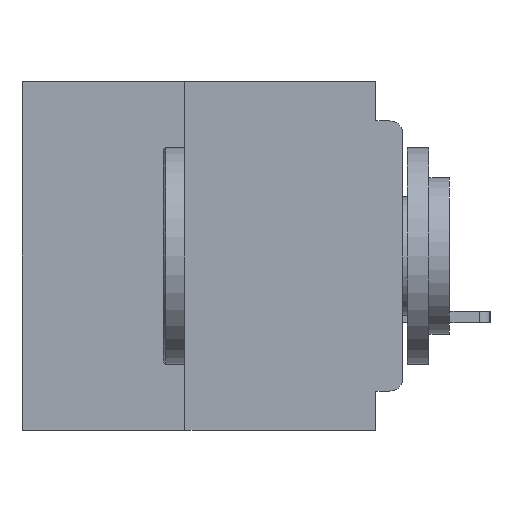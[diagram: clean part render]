
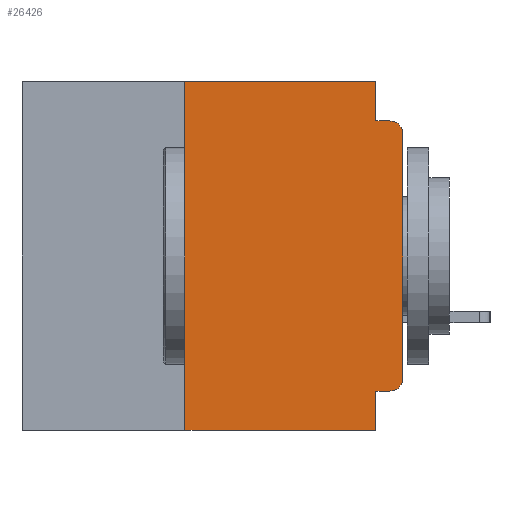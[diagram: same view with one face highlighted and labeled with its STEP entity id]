
A CAD part, left-side view. The second image highlights one B-rep face of the part: STEP entity #26426.
In plain terms, the highlighted planar face has unit normal (-1, 0, 0).
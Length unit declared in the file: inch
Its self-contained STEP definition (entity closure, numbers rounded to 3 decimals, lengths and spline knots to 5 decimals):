
#33 = EDGE_LOOP ( 'NONE', ( #9051, #60994, #26402, #7622, #40816, #59518, #19257, #46271, #60923, #62582 ) ) ;
#771 = DIRECTION ( 'NONE',  ( 0., 0., -1. ) ) ;
#888 = VECTOR ( 'NONE', #58577, 39.37008 ) ;
#1678 = CARTESIAN_POINT ( 'NONE',  ( 0., 0.25, -0.4 ) ) ;
#3356 = DIRECTION ( 'NONE',  ( 0., 1., 0. ) ) ;
#4537 = DIRECTION ( 'NONE',  ( 0., 0., 1. ) ) ;
#5880 = CARTESIAN_POINT ( 'NONE',  ( 0., 0.031, 0. ) ) ;
#7622 = ORIENTED_EDGE ( 'NONE', *, *, #59408, .F. ) ;
#7749 = AXIS2_PLACEMENT_3D ( 'NONE', #62026, #22219, #57303 ) ;
#8075 = VECTOR ( 'NONE', #53399, 39.37008 ) ;
#8453 = CARTESIAN_POINT ( 'NONE',  ( 0., 0.015, -0.045 ) ) ;
#9051 = ORIENTED_EDGE ( 'NONE', *, *, #34646, .T. ) ;
#9626 = VERTEX_POINT ( 'NONE', #39708 ) ;
#11649 = CARTESIAN_POINT ( 'NONE',  ( 0., 0.031, -0.045 ) ) ;
#12040 = PLANE ( 'NONE',  #7749 ) ;
#12617 = VERTEX_POINT ( 'NONE', #48207 ) ;
#12691 = EDGE_CURVE ( 'NONE', #53178, #45963, #41267, .T. ) ;
#13247 = VECTOR ( 'NONE', #771, 39.37008 ) ;
#13794 = CARTESIAN_POINT ( 'NONE',  ( 0., 0.015, -0.06 ) ) ;
#14770 = CARTESIAN_POINT ( 'NONE',  ( 0., 0.25, -0.4 ) ) ;
#16021 = FACE_OUTER_BOUND ( 'NONE', #33, .T. ) ;
#18891 = DIRECTION ( 'NONE',  ( 0., 0., -1. ) ) ;
#19257 = ORIENTED_EDGE ( 'NONE', *, *, #12691, .T. ) ;
#19474 = VERTEX_POINT ( 'NONE', #31330 ) ;
#19723 = DIRECTION ( 'NONE',  ( -1., 0., 0. ) ) ;
#22219 = DIRECTION ( 'NONE',  ( 1., 0., 0. ) ) ;
#22648 = CARTESIAN_POINT ( 'NONE',  ( 0., 0., -0.045 ) ) ;
#22833 = VERTEX_POINT ( 'NONE', #31125 ) ;
#23143 = LINE ( 'NONE', #28608, #34986 ) ;
#23172 = LINE ( 'NONE', #48391, #8075 ) ;
#24656 = LINE ( 'NONE', #22648, #62980 ) ;
#24707 = VERTEX_POINT ( 'NONE', #8453 ) ;
#26339 = CARTESIAN_POINT ( 'NONE',  ( 0., 0., 0. ) ) ;
#26402 = ORIENTED_EDGE ( 'NONE', *, *, #45904, .F. ) ;
#26426 = ADVANCED_FACE ( 'NONE', ( #16021 ), #12040, .F. ) ;
#27227 = CARTESIAN_POINT ( 'NONE',  ( 0., 0., -0.06 ) ) ;
#27704 = EDGE_CURVE ( 'NONE', #39476, #19474, #41979, .T. ) ;
#27709 = DIRECTION ( 'NONE',  ( 0., -1., 0. ) ) ;
#28287 = VECTOR ( 'NONE', #63703, 39.37008 ) ;
#28608 = CARTESIAN_POINT ( 'NONE',  ( 0., 0., -0.355 ) ) ;
#31125 = CARTESIAN_POINT ( 'NONE',  ( 0., 0.031, -0.355 ) ) ;
#31330 = CARTESIAN_POINT ( 'NONE',  ( 0., 0., -0.34 ) ) ;
#33466 = VERTEX_POINT ( 'NONE', #11649 ) ;
#34515 = VECTOR ( 'NONE', #41543, 39.37008 ) ;
#34646 = EDGE_CURVE ( 'NONE', #19474, #50135, #47851, .T. ) ;
#34986 = VECTOR ( 'NONE', #3356, 39.37008 ) ;
#37885 = CARTESIAN_POINT ( 'NONE',  ( 0., 0.031, -0.4 ) ) ;
#39476 = VERTEX_POINT ( 'NONE', #58532 ) ;
#39708 = CARTESIAN_POINT ( 'NONE',  ( 0., 0.25, 0. ) ) ;
#40281 = VECTOR ( 'NONE', #4537, 39.37008 ) ;
#40816 = ORIENTED_EDGE ( 'NONE', *, *, #60432, .F. ) ;
#41267 = LINE ( 'NONE', #53653, #888 ) ;
#41543 = DIRECTION ( 'NONE',  ( 0., 0., 1. ) ) ;
#41979 = CIRCLE ( 'NONE', #50081, 0.015 ) ;
#43113 = CIRCLE ( 'NONE', #58269, 0.015 ) ;
#43427 = LINE ( 'NONE', #14770, #40281 ) ;
#45904 = EDGE_CURVE ( 'NONE', #33466, #24707, #24656, .T. ) ;
#45963 = VERTEX_POINT ( 'NONE', #37885 ) ;
#46271 = ORIENTED_EDGE ( 'NONE', *, *, #48821, .F. ) ;
#47851 = LINE ( 'NONE', #26339, #34515 ) ;
#48207 = CARTESIAN_POINT ( 'NONE',  ( 0., 0.031, 0. ) ) ;
#48391 = CARTESIAN_POINT ( 'NONE',  ( 0., 0.437, 0. ) ) ;
#48821 = EDGE_CURVE ( 'NONE', #22833, #45963, #56508, .T. ) ;
#49045 = DIRECTION ( 'NONE',  ( -1., 0., 0. ) ) ;
#49890 = CARTESIAN_POINT ( 'NONE',  ( 0., 0.015, -0.34 ) ) ;
#50081 = AXIS2_PLACEMENT_3D ( 'NONE', #49890, #19723, #54868 ) ;
#50135 = VERTEX_POINT ( 'NONE', #27227 ) ;
#51590 = EDGE_CURVE ( 'NONE', #39476, #22833, #23143, .T. ) ;
#53026 = EDGE_CURVE ( 'NONE', #53178, #9626, #43427, .T. ) ;
#53178 = VERTEX_POINT ( 'NONE', #1678 ) ;
#53399 = DIRECTION ( 'NONE',  ( 0., -1., 0. ) ) ;
#53405 = LINE ( 'NONE', #5880, #13247 ) ;
#53653 = CARTESIAN_POINT ( 'NONE',  ( 0., 0.437, -0.4 ) ) ;
#54868 = DIRECTION ( 'NONE',  ( 0., 0., -1. ) ) ;
#56508 = LINE ( 'NONE', #58531, #28287 ) ;
#57303 = DIRECTION ( 'NONE',  ( 0., 0., -1. ) ) ;
#58269 = AXIS2_PLACEMENT_3D ( 'NONE', #13794, #49045, #18891 ) ;
#58531 = CARTESIAN_POINT ( 'NONE',  ( 0., 0.031, -0.4 ) ) ;
#58532 = CARTESIAN_POINT ( 'NONE',  ( 0., 0.015, -0.355 ) ) ;
#58577 = DIRECTION ( 'NONE',  ( 0., -1., 0. ) ) ;
#59408 = EDGE_CURVE ( 'NONE', #12617, #33466, #53405, .T. ) ;
#59518 = ORIENTED_EDGE ( 'NONE', *, *, #53026, .F. ) ;
#60432 = EDGE_CURVE ( 'NONE', #9626, #12617, #23172, .T. ) ;
#60923 = ORIENTED_EDGE ( 'NONE', *, *, #51590, .F. ) ;
#60994 = ORIENTED_EDGE ( 'NONE', *, *, #64930, .T. ) ;
#62026 = CARTESIAN_POINT ( 'NONE',  ( 0., 0.437, 0. ) ) ;
#62582 = ORIENTED_EDGE ( 'NONE', *, *, #27704, .T. ) ;
#62980 = VECTOR ( 'NONE', #27709, 39.37008 ) ;
#63703 = DIRECTION ( 'NONE',  ( 0., 0., -1. ) ) ;
#64930 = EDGE_CURVE ( 'NONE', #50135, #24707, #43113, .T. ) ;
